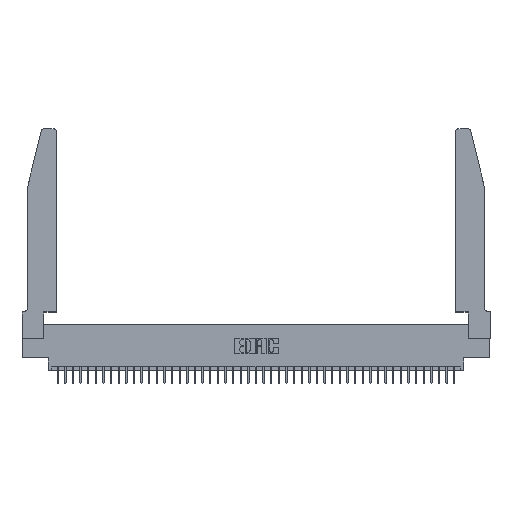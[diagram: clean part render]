
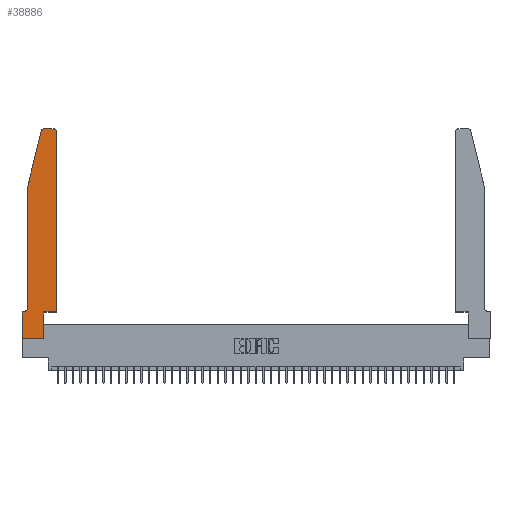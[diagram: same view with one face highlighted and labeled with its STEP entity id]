
A CAD part, top view. The second image highlights one B-rep face of the part: STEP entity #38886.
In plain terms, the highlighted planar face has unit normal (0, 0, 1).
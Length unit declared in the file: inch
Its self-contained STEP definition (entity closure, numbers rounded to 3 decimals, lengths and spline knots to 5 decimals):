
#451 = EDGE_CURVE ( 'NONE', #41261, #16846, #35045, .T. ) ;
#1309 = DIRECTION ( 'NONE',  ( 0., 0., 1. ) ) ;
#1740 = LINE ( 'NONE', #35512, #32756 ) ;
#2054 = VERTEX_POINT ( 'NONE', #41627 ) ;
#2165 = EDGE_CURVE ( 'NONE', #32559, #18358, #25704, .T. ) ;
#2644 = CARTESIAN_POINT ( 'NONE',  ( 0.0755, 0.42, 0.37 ) ) ;
#3047 = ORIENTED_EDGE ( 'NONE', *, *, #8727, .T. ) ;
#3182 = CARTESIAN_POINT ( 'NONE',  ( 0.2865, 0.35, 0.37 ) ) ;
#3385 = DIRECTION ( 'NONE',  ( 1., 0., 0. ) ) ;
#3478 = CARTESIAN_POINT ( 'NONE',  ( 0.4205, 2.75, 0.37 ) ) ;
#4391 = DIRECTION ( 'NONE',  ( 1., 0., 0. ) ) ;
#4658 = ORIENTED_EDGE ( 'NONE', *, *, #36280, .T. ) ;
#5511 = CARTESIAN_POINT ( 'NONE',  ( 0.0755, 0.35, 0.37 ) ) ;
#6296 = ORIENTED_EDGE ( 'NONE', *, *, #14453, .T. ) ;
#7239 = AXIS2_PLACEMENT_3D ( 'NONE', #35379, #27857, #34948 ) ;
#7733 = CARTESIAN_POINT ( 'NONE',  ( 0.284, 2.75, 0.37 ) ) ;
#8180 = CARTESIAN_POINT ( 'NONE',  ( 0., 0.35, 0.37 ) ) ;
#8727 = EDGE_CURVE ( 'NONE', #16846, #38401, #27015, .T. ) ;
#8949 = DIRECTION ( 'NONE',  ( 0., 1., 0. ) ) ;
#9044 = VECTOR ( 'NONE', #33312, 39.37008 ) ;
#9491 = CARTESIAN_POINT ( 'NONE',  ( 0.0755, 2., 0.37 ) ) ;
#9977 = VERTEX_POINT ( 'NONE', #28031 ) ;
#10003 = DIRECTION ( 'NONE',  ( 0., 0., 1. ) ) ;
#10010 = ORIENTED_EDGE ( 'NONE', *, *, #13354, .T. ) ;
#10918 = DIRECTION ( 'NONE',  ( 0., 1., 0. ) ) ;
#11405 = CARTESIAN_POINT ( 'NONE',  ( 0., 0., 0.37 ) ) ;
#11645 = PLANE ( 'NONE',  #32511 ) ;
#12104 = EDGE_LOOP ( 'NONE', ( #12862, #22069, #10010, #6296, #31132, #3047, #4658, #23394, #30577, #18208, #28724, #25185 ) ) ;
#12127 = CARTESIAN_POINT ( 'NONE',  ( 0.284, 2.72, 0.37 ) ) ;
#12862 = ORIENTED_EDGE ( 'NONE', *, *, #17389, .T. ) ;
#13283 = CIRCLE ( 'NONE', #38614, 0.03 ) ;
#13354 = EDGE_CURVE ( 'NONE', #20659, #2054, #28824, .T. ) ;
#13867 = CARTESIAN_POINT ( 'NONE',  ( 0.4505, 0.35, 0.37 ) ) ;
#13868 = CARTESIAN_POINT ( 'NONE',  ( 0.4505, 0.35, 0.37 ) ) ;
#13896 = LINE ( 'NONE', #11405, #33484 ) ;
#14453 = EDGE_CURVE ( 'NONE', #2054, #41261, #27699, .T. ) ;
#15564 = CIRCLE ( 'NONE', #41689, 0.03 ) ;
#15828 = CARTESIAN_POINT ( 'NONE',  ( 0.0755, 2., 0.37 ) ) ;
#15867 = EDGE_CURVE ( 'NONE', #22830, #20659, #15564, .T. ) ;
#16047 = EDGE_CURVE ( 'NONE', #21590, #32559, #13896, .T. ) ;
#16656 = CARTESIAN_POINT ( 'NONE',  ( 0.2865, 0., 0.37 ) ) ;
#16846 = VERTEX_POINT ( 'NONE', #33750 ) ;
#17389 = EDGE_CURVE ( 'NONE', #33235, #22830, #1740, .T. ) ;
#17468 = FACE_OUTER_BOUND ( 'NONE', #12104, .T. ) ;
#18010 = VECTOR ( 'NONE', #3385, 39.37008 ) ;
#18208 = ORIENTED_EDGE ( 'NONE', *, *, #38517, .T. ) ;
#18358 = VERTEX_POINT ( 'NONE', #41066 ) ;
#19852 = LINE ( 'NONE', #34266, #42040 ) ;
#20032 = DIRECTION ( 'NONE',  ( 1., 0., 0. ) ) ;
#20659 = VERTEX_POINT ( 'NONE', #30477 ) ;
#21590 = VERTEX_POINT ( 'NONE', #28969 ) ;
#21880 = DIRECTION ( 'NONE',  ( -1., 0., 0. ) ) ;
#22069 = ORIENTED_EDGE ( 'NONE', *, *, #15867, .T. ) ;
#22274 = DIRECTION ( 'NONE',  ( 1., 0., 0. ) ) ;
#22471 = VECTOR ( 'NONE', #8949, 39.37008 ) ;
#22830 = VERTEX_POINT ( 'NONE', #7733 ) ;
#23394 = ORIENTED_EDGE ( 'NONE', *, *, #16047, .T. ) ;
#25185 = ORIENTED_EDGE ( 'NONE', *, *, #36647, .T. ) ;
#25704 = LINE ( 'NONE', #3182, #22471 ) ;
#27015 = LINE ( 'NONE', #5511, #9044 ) ;
#27029 = DIRECTION ( 'NONE',  ( -0.239, -0.971, 0. ) ) ;
#27699 = LINE ( 'NONE', #15828, #40229 ) ;
#27857 = DIRECTION ( 'NONE',  ( 0., 0., -1. ) ) ;
#28031 = CARTESIAN_POINT ( 'NONE',  ( 0.4505, 2.72, 0.37 ) ) ;
#28724 = ORIENTED_EDGE ( 'NONE', *, *, #38114, .T. ) ;
#28824 = LINE ( 'NONE', #9491, #33747 ) ;
#28833 = LINE ( 'NONE', #13868, #18010 ) ;
#28969 = CARTESIAN_POINT ( 'NONE',  ( 0., 0., 0.37 ) ) ;
#30477 = CARTESIAN_POINT ( 'NONE',  ( 0.25487, 2.72718, 0.37 ) ) ;
#30478 = DIRECTION ( 'NONE',  ( 0., 0., 1. ) ) ;
#30577 = ORIENTED_EDGE ( 'NONE', *, *, #2165, .T. ) ;
#31132 = ORIENTED_EDGE ( 'NONE', *, *, #451, .T. ) ;
#32511 = AXIS2_PLACEMENT_3D ( 'NONE', #8180, #1309, #4391 ) ;
#32559 = VERTEX_POINT ( 'NONE', #16656 ) ;
#32756 = VECTOR ( 'NONE', #21880, 39.37008 ) ;
#32855 = CARTESIAN_POINT ( 'NONE',  ( 0., 0.35, 0.37 ) ) ;
#33235 = VERTEX_POINT ( 'NONE', #3478 ) ;
#33312 = DIRECTION ( 'NONE',  ( -1., 0., 0. ) ) ;
#33484 = VECTOR ( 'NONE', #22274, 39.37008 ) ;
#33747 = VECTOR ( 'NONE', #27029, 39.37008 ) ;
#33750 = CARTESIAN_POINT ( 'NONE',  ( 0.0055, 0.35, 0.37 ) ) ;
#34266 = CARTESIAN_POINT ( 'NONE',  ( 0., 0., 0.37 ) ) ;
#34948 = DIRECTION ( 'NONE',  ( -1., 0., 0. ) ) ;
#35045 = CIRCLE ( 'NONE', #7239, 0.07 ) ;
#35379 = CARTESIAN_POINT ( 'NONE',  ( 0.0055, 0.42, 0.37 ) ) ;
#35512 = CARTESIAN_POINT ( 'NONE',  ( 0.2605, 2.75, 0.37 ) ) ;
#36050 = DIRECTION ( 'NONE',  ( 0., -1., 0. ) ) ;
#36280 = EDGE_CURVE ( 'NONE', #38401, #21590, #19852, .T. ) ;
#36517 = CARTESIAN_POINT ( 'NONE',  ( 0.4505, 0.35, 0.37 ) ) ;
#36647 = EDGE_CURVE ( 'NONE', #9977, #33235, #13283, .T. ) ;
#37836 = DIRECTION ( 'NONE',  ( 1., 0., 0. ) ) ;
#38114 = EDGE_CURVE ( 'NONE', #43641, #9977, #43091, .T. ) ;
#38401 = VERTEX_POINT ( 'NONE', #32855 ) ;
#38517 = EDGE_CURVE ( 'NONE', #18358, #43641, #28833, .T. ) ;
#38614 = AXIS2_PLACEMENT_3D ( 'NONE', #40674, #30478, #20032 ) ;
#38886 = ADVANCED_FACE ( 'NONE', ( #17468 ), #11645, .T. ) ;
#40229 = VECTOR ( 'NONE', #43470, 39.37008 ) ;
#40674 = CARTESIAN_POINT ( 'NONE',  ( 0.4205, 2.72, 0.37 ) ) ;
#41066 = CARTESIAN_POINT ( 'NONE',  ( 0.2865, 0.35, 0.37 ) ) ;
#41261 = VERTEX_POINT ( 'NONE', #2644 ) ;
#41486 = VECTOR ( 'NONE', #10918, 39.37008 ) ;
#41627 = CARTESIAN_POINT ( 'NONE',  ( 0.0755, 2., 0.37 ) ) ;
#41689 = AXIS2_PLACEMENT_3D ( 'NONE', #12127, #10003, #37836 ) ;
#42040 = VECTOR ( 'NONE', #36050, 39.37008 ) ;
#43091 = LINE ( 'NONE', #13867, #41486 ) ;
#43470 = DIRECTION ( 'NONE',  ( 0., -1., 0. ) ) ;
#43641 = VERTEX_POINT ( 'NONE', #36517 ) ;
